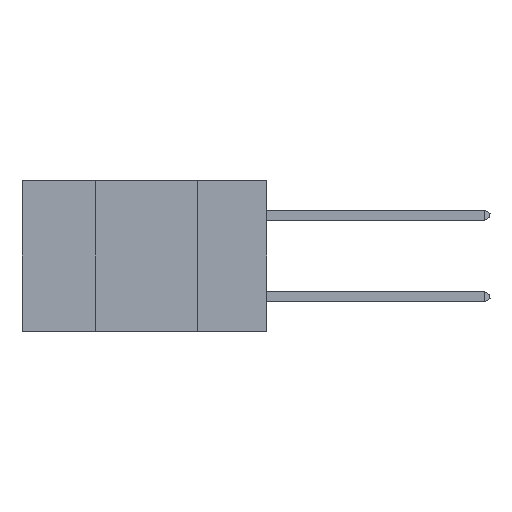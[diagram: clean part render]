
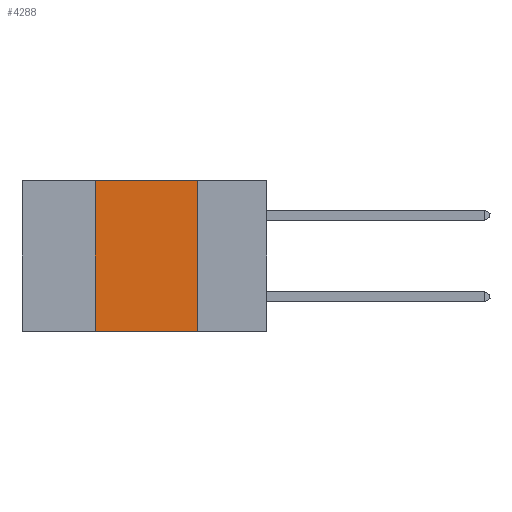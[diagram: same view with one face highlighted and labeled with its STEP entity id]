
A CAD part, left-side view. The second image highlights one B-rep face of the part: STEP entity #4288.
In plain terms, the highlighted planar face has unit normal (-1, 0, 0).
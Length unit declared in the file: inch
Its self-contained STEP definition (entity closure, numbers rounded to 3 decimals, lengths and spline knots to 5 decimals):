
#227 = VERTEX_POINT ( 'NONE', #2235 ) ;
#539 = EDGE_LOOP ( 'NONE', ( #2313, #5409, #7165, #10658 ) ) ;
#1053 = CARTESIAN_POINT ( 'NONE',  ( 0., 0.42, -0.37 ) ) ;
#1174 = CARTESIAN_POINT ( 'NONE',  ( 0., 0.42, 0. ) ) ;
#1672 = FACE_OUTER_BOUND ( 'NONE', #539, .T. ) ;
#2184 = DIRECTION ( 'NONE',  ( 0., 0., 1. ) ) ;
#2235 = CARTESIAN_POINT ( 'NONE',  ( 0., 0.17, 0. ) ) ;
#2313 = ORIENTED_EDGE ( 'NONE', *, *, #2821, .F. ) ;
#2664 = LINE ( 'NONE', #8520, #10235 ) ;
#2821 = EDGE_CURVE ( 'NONE', #227, #10397, #5325, .T. ) ;
#2845 = DIRECTION ( 'NONE',  ( 0., 0., -1. ) ) ;
#3075 = PLANE ( 'NONE',  #12039 ) ;
#3117 = DIRECTION ( 'NONE',  ( 0., 0., -1. ) ) ;
#3298 = VECTOR ( 'NONE', #2184, 39.37008 ) ;
#3964 = EDGE_CURVE ( 'NONE', #11401, #227, #10963, .T. ) ;
#4288 = ADVANCED_FACE ( 'NONE', ( #1672 ), #3075, .F. ) ;
#5325 = LINE ( 'NONE', #6852, #10261 ) ;
#5408 = VECTOR ( 'NONE', #12415, 39.37008 ) ;
#5409 = ORIENTED_EDGE ( 'NONE', *, *, #3964, .F. ) ;
#6073 = CARTESIAN_POINT ( 'NONE',  ( 0., 0.17, -0.37 ) ) ;
#6290 = LINE ( 'NONE', #1174, #3298 ) ;
#6852 = CARTESIAN_POINT ( 'NONE',  ( 0., 0.17, 0. ) ) ;
#7122 = EDGE_CURVE ( 'NONE', #9728, #11401, #6290, .T. ) ;
#7131 = CARTESIAN_POINT ( 'NONE',  ( 0., 0.6, 0. ) ) ;
#7165 = ORIENTED_EDGE ( 'NONE', *, *, #7122, .F. ) ;
#7559 = DIRECTION ( 'NONE',  ( 0., -1., 0. ) ) ;
#8520 = CARTESIAN_POINT ( 'NONE',  ( 0., 0.6, -0.37 ) ) ;
#8557 = CARTESIAN_POINT ( 'NONE',  ( 0., 0.6, 0. ) ) ;
#8560 = CARTESIAN_POINT ( 'NONE',  ( 0., 0.42, 0. ) ) ;
#9056 = DIRECTION ( 'NONE',  ( 1., 0., 0. ) ) ;
#9728 = VERTEX_POINT ( 'NONE', #1053 ) ;
#10235 = VECTOR ( 'NONE', #7559, 39.37008 ) ;
#10261 = VECTOR ( 'NONE', #2845, 39.37008 ) ;
#10397 = VERTEX_POINT ( 'NONE', #6073 ) ;
#10612 = EDGE_CURVE ( 'NONE', #9728, #10397, #2664, .T. ) ;
#10658 = ORIENTED_EDGE ( 'NONE', *, *, #10612, .T. ) ;
#10963 = LINE ( 'NONE', #8557, #5408 ) ;
#11401 = VERTEX_POINT ( 'NONE', #8560 ) ;
#12039 = AXIS2_PLACEMENT_3D ( 'NONE', #7131, #9056, #3117 ) ;
#12415 = DIRECTION ( 'NONE',  ( 0., -1., 0. ) ) ;
